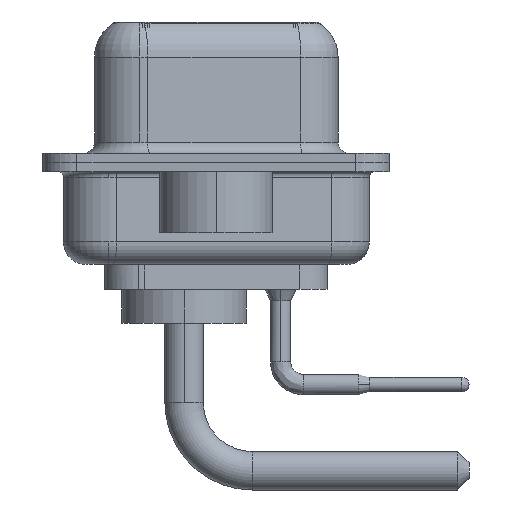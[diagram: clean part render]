
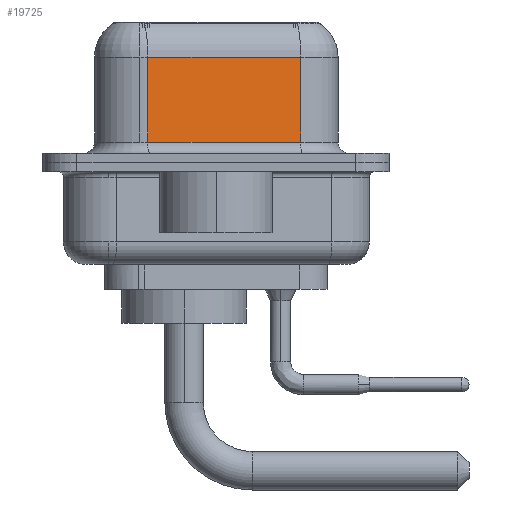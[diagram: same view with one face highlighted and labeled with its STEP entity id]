
A CAD part, left-side view. The second image highlights one B-rep face of the part: STEP entity #19725.
In plain terms, the highlighted planar face has unit normal (-0.985, -0.174, 0).
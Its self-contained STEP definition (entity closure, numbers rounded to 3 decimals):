
#756 = EDGE_LOOP ( 'NONE', ( #2385, #13138, #11368, #11496 ) ) ;
#959 = VECTOR ( 'NONE', #5543, 1000. ) ;
#1283 = DIRECTION ( 'NONE',  ( 0.174, -0.985, 0. ) ) ;
#1477 = VECTOR ( 'NONE', #12031, 1000. ) ;
#1935 = CARTESIAN_POINT ( 'NONE',  ( 5.621, -3.722, 6.4 ) ) ;
#2246 = FACE_OUTER_BOUND ( 'NONE', #756, .T. ) ;
#2385 = ORIENTED_EDGE ( 'NONE', *, *, #2404, .F. ) ;
#2404 = EDGE_CURVE ( 'NONE', #4868, #2946, #5154, .T. ) ;
#2494 = VERTEX_POINT ( 'NONE', #20124 ) ;
#2946 = VERTEX_POINT ( 'NONE', #11691 ) ;
#3584 = VERTEX_POINT ( 'NONE', #7901 ) ;
#4868 = VERTEX_POINT ( 'NONE', #4910 ) ;
#4910 = CARTESIAN_POINT ( 'NONE',  ( 5.621, -3.722, 4.65 ) ) ;
#5154 = LINE ( 'NONE', #6751, #1477 ) ;
#5234 = EDGE_CURVE ( 'NONE', #4868, #3584, #13336, .T. ) ;
#5543 = DIRECTION ( 'NONE',  ( 0., 0., -1. ) ) ;
#5910 = EDGE_CURVE ( 'NONE', #3584, #2494, #10376, .T. ) ;
#6751 = CARTESIAN_POINT ( 'NONE',  ( 5.621, -3.722, 6.4 ) ) ;
#7901 = CARTESIAN_POINT ( 'NONE',  ( 4.43, 3.028, 4.65 ) ) ;
#7940 = VECTOR ( 'NONE', #16368, 1000. ) ;
#10376 = LINE ( 'NONE', #13721, #959 ) ;
#11368 = ORIENTED_EDGE ( 'NONE', *, *, #5910, .T. ) ;
#11496 = ORIENTED_EDGE ( 'NONE', *, *, #16199, .T. ) ;
#11691 = CARTESIAN_POINT ( 'NONE',  ( 5.621, -3.722, 0.9 ) ) ;
#12031 = DIRECTION ( 'NONE',  ( 0., 0., -1. ) ) ;
#12556 = CARTESIAN_POINT ( 'NONE',  ( 5.621, -3.722, 0.9 ) ) ;
#13138 = ORIENTED_EDGE ( 'NONE', *, *, #5234, .T. ) ;
#13336 = LINE ( 'NONE', #19927, #7940 ) ;
#13416 = DIRECTION ( 'NONE',  ( 0.985, 0.174, 0. ) ) ;
#13721 = CARTESIAN_POINT ( 'NONE',  ( 4.43, 3.028, 6.4 ) ) ;
#16199 = EDGE_CURVE ( 'NONE', #2494, #2946, #17326, .T. ) ;
#16368 = DIRECTION ( 'NONE',  ( -0.174, 0.985, 0. ) ) ;
#17193 = DIRECTION ( 'NONE',  ( -0.174, 0.985, 0. ) ) ;
#17326 = LINE ( 'NONE', #12556, #19158 ) ;
#18287 = PLANE ( 'NONE',  #18901 ) ;
#18901 = AXIS2_PLACEMENT_3D ( 'NONE', #1935, #13416, #17193 ) ;
#19158 = VECTOR ( 'NONE', #1283, 1000. ) ;
#19725 = ADVANCED_FACE ( 'NONE', ( #2246 ), #18287, .F. ) ;
#19927 = CARTESIAN_POINT ( 'NONE',  ( 5.621, -3.722, 4.65 ) ) ;
#20124 = CARTESIAN_POINT ( 'NONE',  ( 4.43, 3.028, 0.9 ) ) ;
